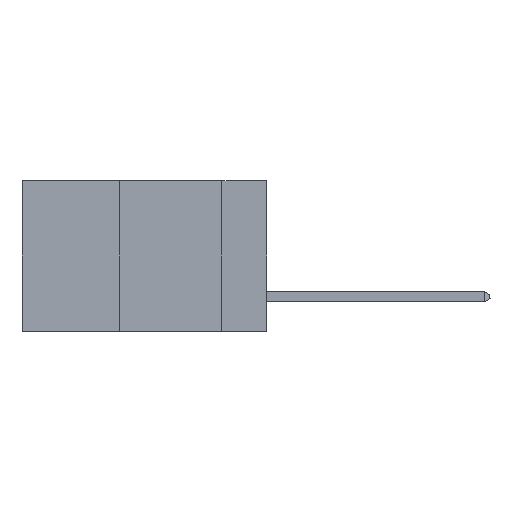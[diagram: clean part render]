
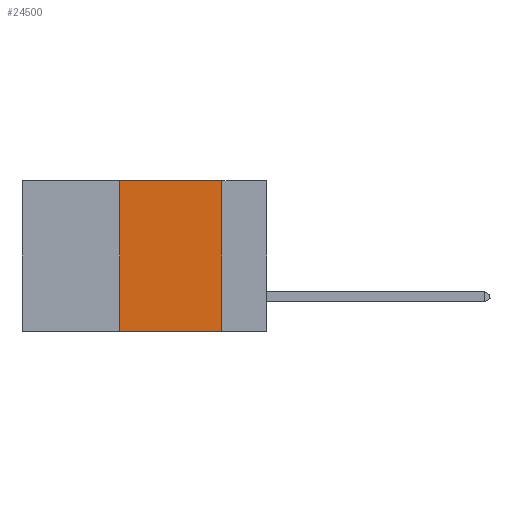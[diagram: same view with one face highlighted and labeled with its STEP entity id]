
A CAD part, left-side view. The second image highlights one B-rep face of the part: STEP entity #24500.
In plain terms, the highlighted planar face has unit normal (-1, 0, 0).
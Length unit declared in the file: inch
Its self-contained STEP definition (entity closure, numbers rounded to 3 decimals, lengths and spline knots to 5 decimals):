
#879 = AXIS2_PLACEMENT_3D ( 'NONE', #11947, #12538, #19177 ) ;
#1818 = ORIENTED_EDGE ( 'NONE', *, *, #10361, .T. ) ;
#1880 = EDGE_LOOP ( 'NONE', ( #30680, #28670, #5514, #1818 ) ) ;
#2594 = VECTOR ( 'NONE', #4584, 39.37008 ) ;
#2681 = PLANE ( 'NONE',  #879 ) ;
#4584 = DIRECTION ( 'NONE',  ( 0., 0., -1. ) ) ;
#5084 = VECTOR ( 'NONE', #40336, 39.37008 ) ;
#5514 = ORIENTED_EDGE ( 'NONE', *, *, #17710, .F. ) ;
#6016 = VECTOR ( 'NONE', #8212, 39.37008 ) ;
#8212 = DIRECTION ( 'NONE',  ( 0., -1., 0. ) ) ;
#8547 = CARTESIAN_POINT ( 'NONE',  ( 0., 0.6, -0.37 ) ) ;
#10361 = EDGE_CURVE ( 'NONE', #32069, #42558, #26174, .T. ) ;
#10662 = CARTESIAN_POINT ( 'NONE',  ( 0., 0.36, 0. ) ) ;
#11842 = DIRECTION ( 'NONE',  ( 0., -1., 0. ) ) ;
#11947 = CARTESIAN_POINT ( 'NONE',  ( 0., 0.6, 0. ) ) ;
#12538 = DIRECTION ( 'NONE',  ( 1., 0., 0. ) ) ;
#15699 = VERTEX_POINT ( 'NONE', #10662 ) ;
#16360 = LINE ( 'NONE', #24391, #6016 ) ;
#17710 = EDGE_CURVE ( 'NONE', #32069, #15699, #27247, .T. ) ;
#19177 = DIRECTION ( 'NONE',  ( 0., 0., -1. ) ) ;
#24391 = CARTESIAN_POINT ( 'NONE',  ( 0., 0.6, 0. ) ) ;
#24500 = ADVANCED_FACE ( 'NONE', ( #33564 ), #2681, .F. ) ;
#24627 = VECTOR ( 'NONE', #11842, 39.37008 ) ;
#25702 = CARTESIAN_POINT ( 'NONE',  ( 0., 0.11, -0.37 ) ) ;
#26174 = LINE ( 'NONE', #8547, #24627 ) ;
#27247 = LINE ( 'NONE', #40531, #5084 ) ;
#28440 = LINE ( 'NONE', #36347, #2594 ) ;
#28670 = ORIENTED_EDGE ( 'NONE', *, *, #29099, .F. ) ;
#29099 = EDGE_CURVE ( 'NONE', #15699, #41625, #16360, .T. ) ;
#30680 = ORIENTED_EDGE ( 'NONE', *, *, #32239, .F. ) ;
#32069 = VERTEX_POINT ( 'NONE', #35675 ) ;
#32239 = EDGE_CURVE ( 'NONE', #41625, #42558, #28440, .T. ) ;
#33564 = FACE_OUTER_BOUND ( 'NONE', #1880, .T. ) ;
#35675 = CARTESIAN_POINT ( 'NONE',  ( 0., 0.36, -0.37 ) ) ;
#36347 = CARTESIAN_POINT ( 'NONE',  ( 0., 0.11, 0. ) ) ;
#40336 = DIRECTION ( 'NONE',  ( 0., 0., 1. ) ) ;
#40531 = CARTESIAN_POINT ( 'NONE',  ( 0., 0.36, 0. ) ) ;
#41625 = VERTEX_POINT ( 'NONE', #42069 ) ;
#42069 = CARTESIAN_POINT ( 'NONE',  ( 0., 0.11, 0. ) ) ;
#42558 = VERTEX_POINT ( 'NONE', #25702 ) ;
